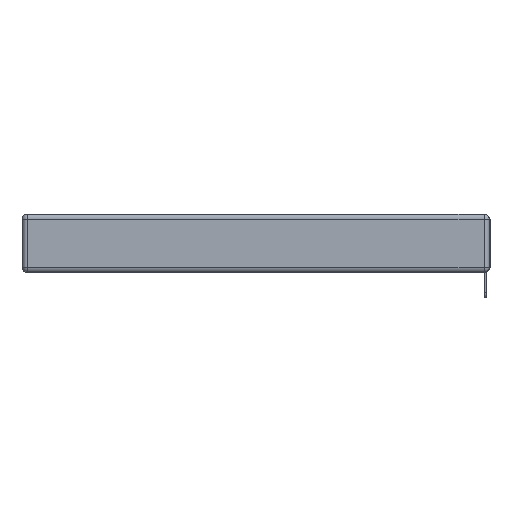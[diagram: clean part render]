
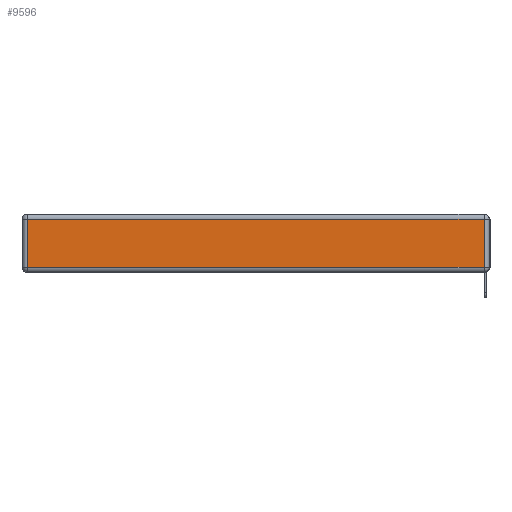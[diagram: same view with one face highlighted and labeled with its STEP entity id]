
A CAD part, left-side view. The second image highlights one B-rep face of the part: STEP entity #9596.
In plain terms, the highlighted planar face has unit normal (-1, 0, 0).
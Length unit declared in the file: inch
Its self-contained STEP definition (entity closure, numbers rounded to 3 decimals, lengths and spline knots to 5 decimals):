
#757 = LINE ( 'NONE', #8011, #21375 ) ;
#1354 = DIRECTION ( 'NONE',  ( 0., 1., 0. ) ) ;
#1652 = DIRECTION ( 'NONE',  ( 0., 0., 1. ) ) ;
#3242 = VERTEX_POINT ( 'NONE', #27584 ) ;
#4063 = VECTOR ( 'NONE', #1354, 39.37008 ) ;
#5130 = PLANE ( 'NONE',  #16059 ) ;
#5955 = DIRECTION ( 'NONE',  ( 0., 0., -1. ) ) ;
#6279 = VERTEX_POINT ( 'NONE', #21669 ) ;
#6304 = VERTEX_POINT ( 'NONE', #8515 ) ;
#7360 = CARTESIAN_POINT ( 'NONE',  ( 0., 0., -0.343 ) ) ;
#7607 = ORIENTED_EDGE ( 'NONE', *, *, #18097, .T. ) ;
#8011 = CARTESIAN_POINT ( 'NONE',  ( 0., 2.72, -0.343 ) ) ;
#8515 = CARTESIAN_POINT ( 'NONE',  ( 0., 2.72, -0.313 ) ) ;
#9596 = ADVANCED_FACE ( 'NONE', ( #27020 ), #5130, .T. ) ;
#12209 = ORIENTED_EDGE ( 'NONE', *, *, #21363, .T. ) ;
#14438 = CARTESIAN_POINT ( 'NONE',  ( 0., 0.03, -0.343 ) ) ;
#15050 = ORIENTED_EDGE ( 'NONE', *, *, #16980, .T. ) ;
#15696 = VECTOR ( 'NONE', #17736, 39.37008 ) ;
#16059 = AXIS2_PLACEMENT_3D ( 'NONE', #7360, #20617, #24473 ) ;
#16152 = CARTESIAN_POINT ( 'NONE',  ( 0., 2.75, -0.03 ) ) ;
#16217 = LINE ( 'NONE', #16152, #4063 ) ;
#16980 = EDGE_CURVE ( 'NONE', #6279, #3242, #25226, .T. ) ;
#17736 = DIRECTION ( 'NONE',  ( 0., -1., 0. ) ) ;
#18097 = EDGE_CURVE ( 'NONE', #6304, #6279, #18749, .T. ) ;
#18749 = LINE ( 'NONE', #26407, #15696 ) ;
#20201 = EDGE_CURVE ( 'NONE', #22368, #6304, #757, .T. ) ;
#20617 = DIRECTION ( 'NONE',  ( -1., 0., 0. ) ) ;
#21363 = EDGE_CURVE ( 'NONE', #3242, #22368, #16217, .T. ) ;
#21375 = VECTOR ( 'NONE', #5955, 39.37008 ) ;
#21669 = CARTESIAN_POINT ( 'NONE',  ( 0., 0.03, -0.313 ) ) ;
#22368 = VERTEX_POINT ( 'NONE', #23551 ) ;
#23537 = VECTOR ( 'NONE', #1652, 39.37008 ) ;
#23551 = CARTESIAN_POINT ( 'NONE',  ( 0., 2.72, -0.03 ) ) ;
#23720 = EDGE_LOOP ( 'NONE', ( #7607, #15050, #12209, #24606 ) ) ;
#24473 = DIRECTION ( 'NONE',  ( 0., 0., 1. ) ) ;
#24606 = ORIENTED_EDGE ( 'NONE', *, *, #20201, .T. ) ;
#25226 = LINE ( 'NONE', #14438, #23537 ) ;
#26407 = CARTESIAN_POINT ( 'NONE',  ( 0., 0., -0.313 ) ) ;
#27020 = FACE_OUTER_BOUND ( 'NONE', #23720, .T. ) ;
#27584 = CARTESIAN_POINT ( 'NONE',  ( 0., 0.03, -0.03 ) ) ;
